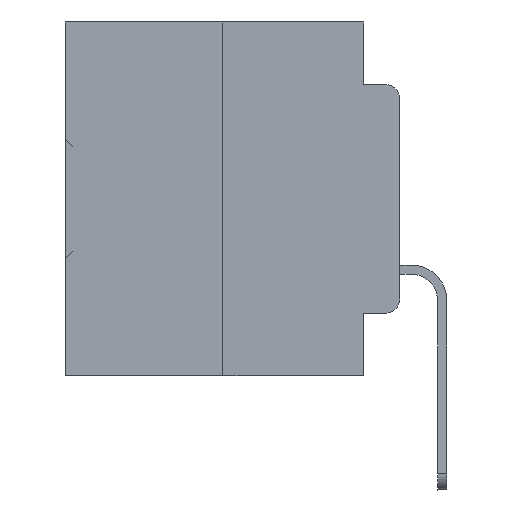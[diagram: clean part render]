
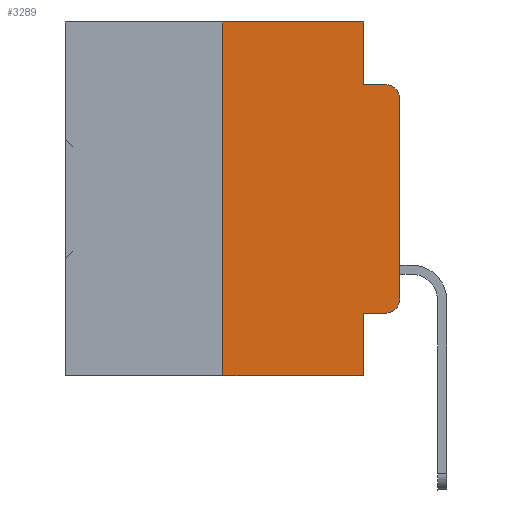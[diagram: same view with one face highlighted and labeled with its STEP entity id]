
A CAD part, left-side view. The second image highlights one B-rep face of the part: STEP entity #3289.
In plain terms, the highlighted planar face has unit normal (-1, 0, 0).
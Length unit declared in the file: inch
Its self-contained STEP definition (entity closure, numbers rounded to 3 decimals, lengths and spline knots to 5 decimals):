
#1212 = CARTESIAN_POINT ( 'NONE',  ( 0., 0.02, -0.3915 ) ) ;
#2781 = DIRECTION ( 'NONE',  ( 0., -1., 0. ) ) ;
#2832 = EDGE_CURVE ( 'NONE', #18909, #28412, #7217, .T. ) ;
#3289 = ADVANCED_FACE ( 'NONE', ( #3622 ), #23967, .F. ) ;
#3622 = FACE_OUTER_BOUND ( 'NONE', #19721, .T. ) ;
#3667 = DIRECTION ( 'NONE',  ( 0., 0., -1. ) ) ;
#4771 = DIRECTION ( 'NONE',  ( 0., 0., 1. ) ) ;
#4901 = VECTOR ( 'NONE', #27034, 39.37008 ) ;
#5601 = CARTESIAN_POINT ( 'NONE',  ( 0., 0.051, -0.0885 ) ) ;
#5891 = EDGE_CURVE ( 'NONE', #21284, #28412, #34795, .T. ) ;
#6337 = ORIENTED_EDGE ( 'NONE', *, *, #30858, .T. ) ;
#6469 = DIRECTION ( 'NONE',  ( 0., 0., -1. ) ) ;
#6558 = CARTESIAN_POINT ( 'NONE',  ( 0., 0.051, -0.0885 ) ) ;
#6887 = VERTEX_POINT ( 'NONE', #9949 ) ;
#7056 = VECTOR ( 'NONE', #12472, 39.37008 ) ;
#7217 = LINE ( 'NONE', #21371, #4901 ) ;
#7230 = VECTOR ( 'NONE', #19158, 39.37008 ) ;
#7305 = LINE ( 'NONE', #21447, #16619 ) ;
#7433 = VECTOR ( 'NONE', #2781, 39.37008 ) ;
#7855 = CARTESIAN_POINT ( 'NONE',  ( 0., 0., -0.3915 ) ) ;
#8353 = CIRCLE ( 'NONE', #8946, 0.02 ) ;
#8417 = EDGE_CURVE ( 'NONE', #21284, #23865, #25020, .T. ) ;
#8873 = ORIENTED_EDGE ( 'NONE', *, *, #5891, .T. ) ;
#8946 = AXIS2_PLACEMENT_3D ( 'NONE', #1212, #24197, #3667 ) ;
#9317 = LINE ( 'NONE', #27010, #10470 ) ;
#9327 = CARTESIAN_POINT ( 'NONE',  ( 0., 0.051, -0.5 ) ) ;
#9475 = CARTESIAN_POINT ( 'NONE',  ( 0., 0.473, 0. ) ) ;
#9780 = DIRECTION ( 'NONE',  ( 0., -1., 0. ) ) ;
#9899 = LINE ( 'NONE', #30609, #13941 ) ;
#9949 = CARTESIAN_POINT ( 'NONE',  ( 0., 0.051, 0. ) ) ;
#10470 = VECTOR ( 'NONE', #6469, 39.37008 ) ;
#10706 = VERTEX_POINT ( 'NONE', #7855 ) ;
#10973 = DIRECTION ( 'NONE',  ( 0., 0., -1. ) ) ;
#12391 = ORIENTED_EDGE ( 'NONE', *, *, #30583, .F. ) ;
#12472 = DIRECTION ( 'NONE',  ( 0., -1., 0. ) ) ;
#13793 = CARTESIAN_POINT ( 'NONE',  ( 0., 0.02, -0.1085 ) ) ;
#13941 = VECTOR ( 'NONE', #4771, 39.37008 ) ;
#14929 = VECTOR ( 'NONE', #17967, 39.37008 ) ;
#15138 = CARTESIAN_POINT ( 'NONE',  ( 0., 0.473, 0. ) ) ;
#15807 = VERTEX_POINT ( 'NONE', #18056 ) ;
#16619 = VECTOR ( 'NONE', #9780, 39.37008 ) ;
#16638 = ORIENTED_EDGE ( 'NONE', *, *, #8417, .F. ) ;
#17825 = CARTESIAN_POINT ( 'NONE',  ( 0., 0.25, 0. ) ) ;
#17934 = EDGE_CURVE ( 'NONE', #6887, #30369, #9317, .T. ) ;
#17967 = DIRECTION ( 'NONE',  ( 0., -1., 0. ) ) ;
#18056 = CARTESIAN_POINT ( 'NONE',  ( 0., 0., -0.1085 ) ) ;
#18909 = VERTEX_POINT ( 'NONE', #36644 ) ;
#19158 = DIRECTION ( 'NONE',  ( 0., 0., 1. ) ) ;
#19721 = EDGE_LOOP ( 'NONE', ( #26180, #6337, #12391, #29908, #31449, #16638, #8873, #25979, #20524, #24396 ) ) ;
#20524 = ORIENTED_EDGE ( 'NONE', *, *, #32915, .T. ) ;
#21284 = VERTEX_POINT ( 'NONE', #29037 ) ;
#21371 = CARTESIAN_POINT ( 'NONE',  ( 0., 0.051, 0. ) ) ;
#21447 = CARTESIAN_POINT ( 'NONE',  ( 0., 0.051, -0.4115 ) ) ;
#22458 = EDGE_CURVE ( 'NONE', #23865, #6887, #23613, .T. ) ;
#23188 = VERTEX_POINT ( 'NONE', #29958 ) ;
#23613 = LINE ( 'NONE', #9475, #7056 ) ;
#23617 = DIRECTION ( 'NONE',  ( 1., 0., 0. ) ) ;
#23835 = VERTEX_POINT ( 'NONE', #34817 ) ;
#23865 = VERTEX_POINT ( 'NONE', #17825 ) ;
#23958 = EDGE_CURVE ( 'NONE', #23188, #10706, #8353, .T. ) ;
#23967 = PLANE ( 'NONE',  #27718 ) ;
#24197 = DIRECTION ( 'NONE',  ( -1., 0., 0. ) ) ;
#24396 = ORIENTED_EDGE ( 'NONE', *, *, #23958, .T. ) ;
#25020 = LINE ( 'NONE', #33533, #7230 ) ;
#25979 = ORIENTED_EDGE ( 'NONE', *, *, #2832, .F. ) ;
#26180 = ORIENTED_EDGE ( 'NONE', *, *, #26889, .T. ) ;
#26638 = DIRECTION ( 'NONE',  ( 0., 0., -1. ) ) ;
#26889 = EDGE_CURVE ( 'NONE', #10706, #15807, #9899, .T. ) ;
#27010 = CARTESIAN_POINT ( 'NONE',  ( 0., 0.051, 0. ) ) ;
#27034 = DIRECTION ( 'NONE',  ( 0., 0., -1. ) ) ;
#27718 = AXIS2_PLACEMENT_3D ( 'NONE', #15138, #23617, #26638 ) ;
#28412 = VERTEX_POINT ( 'NONE', #9327 ) ;
#29037 = CARTESIAN_POINT ( 'NONE',  ( 0., 0.25, -0.5 ) ) ;
#29908 = ORIENTED_EDGE ( 'NONE', *, *, #17934, .F. ) ;
#29958 = CARTESIAN_POINT ( 'NONE',  ( 0., 0.02, -0.4115 ) ) ;
#30369 = VERTEX_POINT ( 'NONE', #6558 ) ;
#30583 = EDGE_CURVE ( 'NONE', #30369, #23835, #34467, .T. ) ;
#30609 = CARTESIAN_POINT ( 'NONE',  ( 0., 0., 0. ) ) ;
#30858 = EDGE_CURVE ( 'NONE', #15807, #23835, #33383, .T. ) ;
#31449 = ORIENTED_EDGE ( 'NONE', *, *, #22458, .F. ) ;
#31767 = CARTESIAN_POINT ( 'NONE',  ( 0., 0.473, -0.5 ) ) ;
#32915 = EDGE_CURVE ( 'NONE', #18909, #23188, #7305, .T. ) ;
#33383 = CIRCLE ( 'NONE', #33989, 0.02 ) ;
#33441 = DIRECTION ( 'NONE',  ( -1., 0., 0. ) ) ;
#33533 = CARTESIAN_POINT ( 'NONE',  ( 0., 0.25, 0. ) ) ;
#33989 = AXIS2_PLACEMENT_3D ( 'NONE', #13793, #33441, #10973 ) ;
#34467 = LINE ( 'NONE', #5601, #7433 ) ;
#34795 = LINE ( 'NONE', #31767, #14929 ) ;
#34817 = CARTESIAN_POINT ( 'NONE',  ( 0., 0.02, -0.0885 ) ) ;
#36644 = CARTESIAN_POINT ( 'NONE',  ( 0., 0.051, -0.4115 ) ) ;
